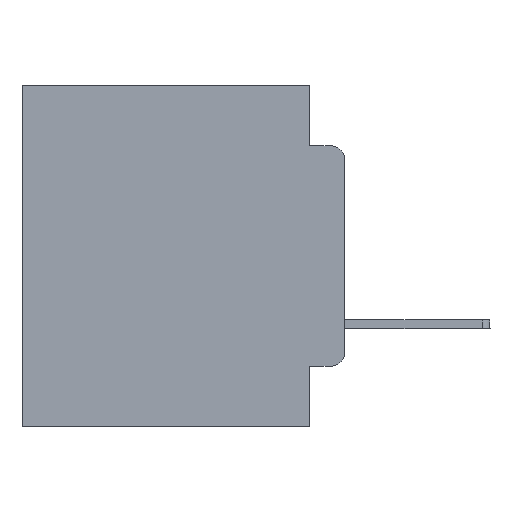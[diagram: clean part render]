
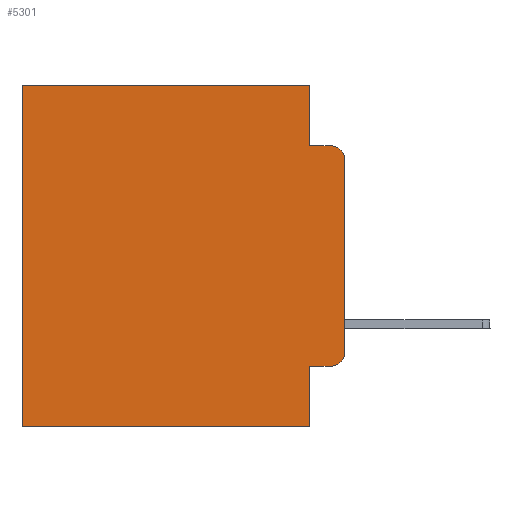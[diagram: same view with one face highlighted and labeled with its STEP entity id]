
A CAD part, left-side view. The second image highlights one B-rep face of the part: STEP entity #5301.
In plain terms, the highlighted planar face has unit normal (-1, 0, 0).
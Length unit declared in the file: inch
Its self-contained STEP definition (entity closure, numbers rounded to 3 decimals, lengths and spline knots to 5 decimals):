
#24 = LINE ( 'NONE', #15892, #14291 ) ;
#573 = EDGE_CURVE ( 'NONE', #5003, #19404, #24, .T. ) ;
#745 = ORIENTED_EDGE ( 'NONE', *, *, #12852, .T. ) ;
#898 = CARTESIAN_POINT ( 'NONE',  ( 0.298, 0.051, -0.4115 ) ) ;
#1051 = VERTEX_POINT ( 'NONE', #8031 ) ;
#1743 = EDGE_CURVE ( 'NONE', #5437, #21563, #20123, .T. ) ;
#2064 = DIRECTION ( 'NONE',  ( 0., 0., -1. ) ) ;
#2190 = EDGE_CURVE ( 'NONE', #19404, #17388, #15111, .T. ) ;
#2444 = VECTOR ( 'NONE', #26890, 39.37008 ) ;
#2712 = ORIENTED_EDGE ( 'NONE', *, *, #18726, .F. ) ;
#3647 = EDGE_LOOP ( 'NONE', ( #20760, #16647, #11400, #2712, #26442, #4606, #20107, #18618, #745, #11837 ) ) ;
#3711 = CIRCLE ( 'NONE', #6693, 0.02 ) ;
#4384 = VERTEX_POINT ( 'NONE', #23203 ) ;
#4606 = ORIENTED_EDGE ( 'NONE', *, *, #6224, .T. ) ;
#5003 = VERTEX_POINT ( 'NONE', #5967 ) ;
#5301 = ADVANCED_FACE ( 'NONE', ( #25695 ), #22320, .F. ) ;
#5437 = VERTEX_POINT ( 'NONE', #8397 ) ;
#5438 = CARTESIAN_POINT ( 'NONE',  ( 0.298, 0.02, -0.1085 ) ) ;
#5606 = DIRECTION ( 'NONE',  ( 0., 0., -1. ) ) ;
#5967 = CARTESIAN_POINT ( 'NONE',  ( 0.298, 0.051, -0.4115 ) ) ;
#6224 = EDGE_CURVE ( 'NONE', #10742, #17388, #8052, .T. ) ;
#6693 = AXIS2_PLACEMENT_3D ( 'NONE', #5438, #15859, #5606 ) ;
#7053 = CARTESIAN_POINT ( 'NONE',  ( 0.298, 0.473, -0.5 ) ) ;
#8031 = CARTESIAN_POINT ( 'NONE',  ( 0.298, 0.051, -0.0885 ) ) ;
#8052 = LINE ( 'NONE', #20863, #11319 ) ;
#8397 = CARTESIAN_POINT ( 'NONE',  ( 0.298, 0.02, -0.4115 ) ) ;
#9889 = CARTESIAN_POINT ( 'NONE',  ( 0.298, 0., -0.5 ) ) ;
#9890 = CARTESIAN_POINT ( 'NONE',  ( 0.298, 0., 0. ) ) ;
#10030 = LINE ( 'NONE', #15622, #25958 ) ;
#10251 = CARTESIAN_POINT ( 'NONE',  ( 0.298, 0.051, 0. ) ) ;
#10742 = VERTEX_POINT ( 'NONE', #13384 ) ;
#11010 = CARTESIAN_POINT ( 'NONE',  ( 0.298, 0., -0.3915 ) ) ;
#11319 = VECTOR ( 'NONE', #19066, 39.37008 ) ;
#11383 = CARTESIAN_POINT ( 'NONE',  ( 0.298, 0., 0. ) ) ;
#11400 = ORIENTED_EDGE ( 'NONE', *, *, #13736, .F. ) ;
#11837 = ORIENTED_EDGE ( 'NONE', *, *, #1743, .T. ) ;
#12704 = LINE ( 'NONE', #18861, #16641 ) ;
#12852 = EDGE_CURVE ( 'NONE', #5003, #5437, #14635, .T. ) ;
#13384 = CARTESIAN_POINT ( 'NONE',  ( 0.298, 0.473, 0. ) ) ;
#13599 = DIRECTION ( 'NONE',  ( -1., 0., 0. ) ) ;
#13736 = EDGE_CURVE ( 'NONE', #1051, #4384, #10030, .T. ) ;
#13876 = DIRECTION ( 'NONE',  ( 1., 0., 0. ) ) ;
#14291 = VECTOR ( 'NONE', #24503, 39.37008 ) ;
#14635 = LINE ( 'NONE', #898, #26017 ) ;
#14775 = LINE ( 'NONE', #11383, #2444 ) ;
#14942 = DIRECTION ( 'NONE',  ( 0., 0., -1. ) ) ;
#15111 = LINE ( 'NONE', #9889, #16062 ) ;
#15614 = DIRECTION ( 'NONE',  ( 0., 0., -1. ) ) ;
#15622 = CARTESIAN_POINT ( 'NONE',  ( 0.298, 0.051, -0.0885 ) ) ;
#15859 = DIRECTION ( 'NONE',  ( -1., 0., 0. ) ) ;
#15892 = CARTESIAN_POINT ( 'NONE',  ( 0.298, 0.051, 0. ) ) ;
#16062 = VECTOR ( 'NONE', #20352, 39.37008 ) ;
#16641 = VECTOR ( 'NONE', #14942, 39.37008 ) ;
#16647 = ORIENTED_EDGE ( 'NONE', *, *, #19459, .T. ) ;
#16838 = CARTESIAN_POINT ( 'NONE',  ( 0.298, 0.051, 0. ) ) ;
#17034 = CARTESIAN_POINT ( 'NONE',  ( 0.298, 0.051, -0.5 ) ) ;
#17388 = VERTEX_POINT ( 'NONE', #7053 ) ;
#18406 = VERTEX_POINT ( 'NONE', #25209 ) ;
#18618 = ORIENTED_EDGE ( 'NONE', *, *, #573, .F. ) ;
#18726 = EDGE_CURVE ( 'NONE', #22194, #1051, #21587, .T. ) ;
#18861 = CARTESIAN_POINT ( 'NONE',  ( 0.298, 0., 0. ) ) ;
#19066 = DIRECTION ( 'NONE',  ( 0., 0., -1. ) ) ;
#19404 = VERTEX_POINT ( 'NONE', #17034 ) ;
#19450 = DIRECTION ( 'NONE',  ( 0., -1., 0. ) ) ;
#19459 = EDGE_CURVE ( 'NONE', #18406, #4384, #3711, .T. ) ;
#20107 = ORIENTED_EDGE ( 'NONE', *, *, #2190, .F. ) ;
#20123 = CIRCLE ( 'NONE', #24471, 0.02 ) ;
#20352 = DIRECTION ( 'NONE',  ( 0., 1., 0. ) ) ;
#20760 = ORIENTED_EDGE ( 'NONE', *, *, #24782, .F. ) ;
#20863 = CARTESIAN_POINT ( 'NONE',  ( 0.298, 0.473, 0. ) ) ;
#21563 = VERTEX_POINT ( 'NONE', #11010 ) ;
#21587 = LINE ( 'NONE', #16838, #22227 ) ;
#21901 = DIRECTION ( 'NONE',  ( 0., -1., 0. ) ) ;
#22194 = VERTEX_POINT ( 'NONE', #10251 ) ;
#22227 = VECTOR ( 'NONE', #2064, 39.37008 ) ;
#22320 = PLANE ( 'NONE',  #22653 ) ;
#22653 = AXIS2_PLACEMENT_3D ( 'NONE', #9890, #13876, #24402 ) ;
#23203 = CARTESIAN_POINT ( 'NONE',  ( 0.298, 0.02, -0.0885 ) ) ;
#23456 = EDGE_CURVE ( 'NONE', #22194, #10742, #14775, .T. ) ;
#23785 = CARTESIAN_POINT ( 'NONE',  ( 0.298, 0.02, -0.3915 ) ) ;
#24402 = DIRECTION ( 'NONE',  ( 0., 0., -1. ) ) ;
#24471 = AXIS2_PLACEMENT_3D ( 'NONE', #23785, #13599, #15614 ) ;
#24503 = DIRECTION ( 'NONE',  ( 0., 0., -1. ) ) ;
#24782 = EDGE_CURVE ( 'NONE', #18406, #21563, #12704, .T. ) ;
#25209 = CARTESIAN_POINT ( 'NONE',  ( 0.298, 0., -0.1085 ) ) ;
#25695 = FACE_OUTER_BOUND ( 'NONE', #3647, .T. ) ;
#25958 = VECTOR ( 'NONE', #21901, 39.37008 ) ;
#26017 = VECTOR ( 'NONE', #19450, 39.37008 ) ;
#26442 = ORIENTED_EDGE ( 'NONE', *, *, #23456, .T. ) ;
#26890 = DIRECTION ( 'NONE',  ( 0., 1., 0. ) ) ;
